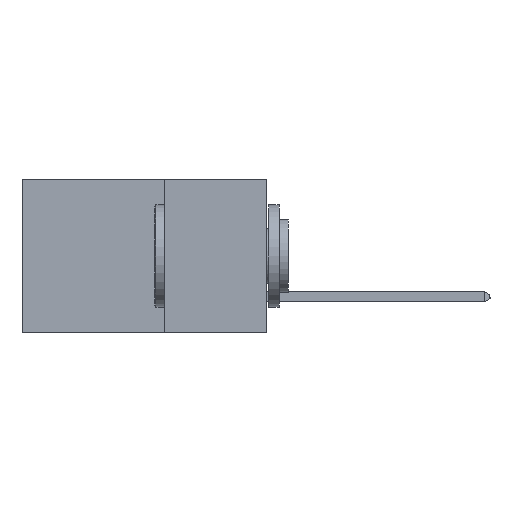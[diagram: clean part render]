
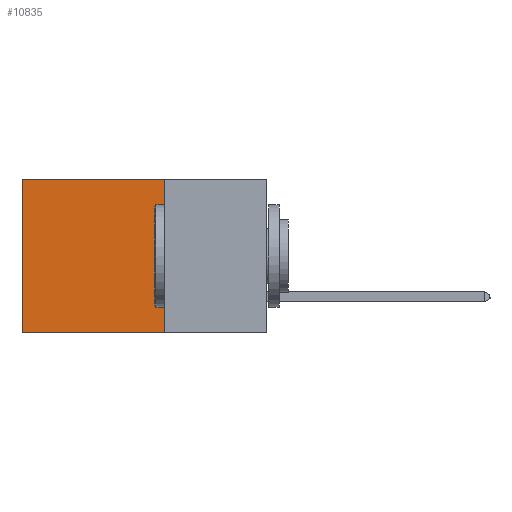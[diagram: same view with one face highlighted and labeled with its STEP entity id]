
A CAD part, left-side view. The second image highlights one B-rep face of the part: STEP entity #10835.
In plain terms, the highlighted planar face has unit normal (-1, 0, 0).
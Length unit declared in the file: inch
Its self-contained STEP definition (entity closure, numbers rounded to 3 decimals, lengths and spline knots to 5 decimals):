
#889 = ORIENTED_EDGE ( 'NONE', *, *, #4357, .T. ) ;
#1279 = EDGE_CURVE ( 'NONE', #3130, #3308, #8103, .T. ) ;
#1307 = CARTESIAN_POINT ( 'NONE',  ( 0.2875, 0.6, -0.375 ) ) ;
#1775 = DIRECTION ( 'NONE',  ( 1., 0., 0. ) ) ;
#2040 = VECTOR ( 'NONE', #11948, 39.37008 ) ;
#2046 = DIRECTION ( 'NONE',  ( 0., 1., 0. ) ) ;
#2690 = VECTOR ( 'NONE', #5634, 39.37008 ) ;
#3090 = LINE ( 'NONE', #6172, #13655 ) ;
#3130 = VERTEX_POINT ( 'NONE', #8632 ) ;
#3242 = EDGE_CURVE ( 'NONE', #3308, #12654, #9975, .T. ) ;
#3308 = VERTEX_POINT ( 'NONE', #4424 ) ;
#3543 = EDGE_CURVE ( 'NONE', #3130, #13822, #3090, .T. ) ;
#4357 = EDGE_CURVE ( 'NONE', #13822, #12654, #8576, .T. ) ;
#4424 = CARTESIAN_POINT ( 'NONE',  ( 0.2875, 0.25, -0.375 ) ) ;
#4952 = CARTESIAN_POINT ( 'NONE',  ( 0.2875, 0.25, -0.375 ) ) ;
#5634 = DIRECTION ( 'NONE',  ( 0., 1., 0. ) ) ;
#5766 = PLANE ( 'NONE',  #9608 ) ;
#6076 = VECTOR ( 'NONE', #8171, 39.37008 ) ;
#6172 = CARTESIAN_POINT ( 'NONE',  ( 0.2875, 0.25, 0. ) ) ;
#7244 = CARTESIAN_POINT ( 'NONE',  ( 0.2875, 0.6, 0. ) ) ;
#8103 = LINE ( 'NONE', #4952, #6076 ) ;
#8171 = DIRECTION ( 'NONE',  ( 0., 0., -1. ) ) ;
#8576 = LINE ( 'NONE', #1307, #2040 ) ;
#8632 = CARTESIAN_POINT ( 'NONE',  ( 0.2875, 0.25, 0. ) ) ;
#9593 = EDGE_LOOP ( 'NONE', ( #889, #13741, #12406, #10970 ) ) ;
#9608 = AXIS2_PLACEMENT_3D ( 'NONE', #10040, #1775, #11155 ) ;
#9917 = FACE_OUTER_BOUND ( 'NONE', #9593, .T. ) ;
#9975 = LINE ( 'NONE', #11091, #2690 ) ;
#10040 = CARTESIAN_POINT ( 'NONE',  ( 0.2875, 0.25, -0.375 ) ) ;
#10100 = CARTESIAN_POINT ( 'NONE',  ( 0.2875, 0.6, -0.375 ) ) ;
#10835 = ADVANCED_FACE ( 'NONE', ( #9917 ), #5766, .F. ) ;
#10970 = ORIENTED_EDGE ( 'NONE', *, *, #3543, .T. ) ;
#11091 = CARTESIAN_POINT ( 'NONE',  ( 0.2875, 0.25, -0.375 ) ) ;
#11155 = DIRECTION ( 'NONE',  ( 0., 0., -1. ) ) ;
#11948 = DIRECTION ( 'NONE',  ( 0., 0., -1. ) ) ;
#12406 = ORIENTED_EDGE ( 'NONE', *, *, #1279, .F. ) ;
#12654 = VERTEX_POINT ( 'NONE', #10100 ) ;
#13655 = VECTOR ( 'NONE', #2046, 39.37008 ) ;
#13741 = ORIENTED_EDGE ( 'NONE', *, *, #3242, .F. ) ;
#13822 = VERTEX_POINT ( 'NONE', #7244 ) ;
